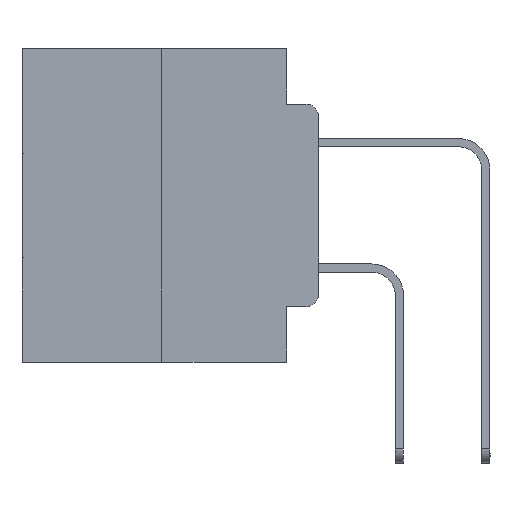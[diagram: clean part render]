
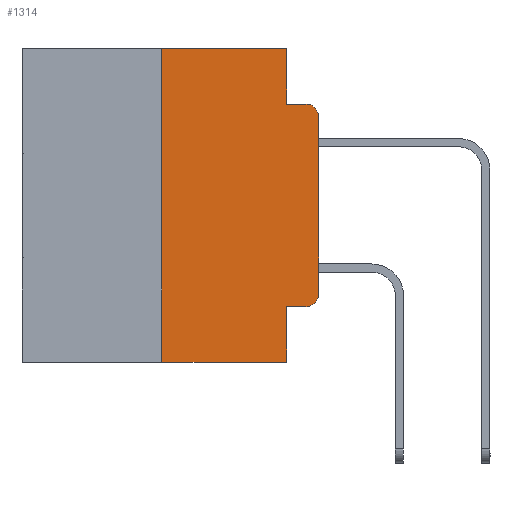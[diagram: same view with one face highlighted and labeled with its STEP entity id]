
A CAD part, left-side view. The second image highlights one B-rep face of the part: STEP entity #1314.
In plain terms, the highlighted planar face has unit normal (-1, 0, 0).
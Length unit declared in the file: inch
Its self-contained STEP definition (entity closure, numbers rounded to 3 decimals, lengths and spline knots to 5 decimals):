
#686 = VECTOR ( 'NONE', #9635, 39.37008 ) ;
#1071 = EDGE_LOOP ( 'NONE', ( #18724, #27887, #17250, #8662, #7042, #16825, #24293, #7595, #14695, #12281 ) ) ;
#1314 = ADVANCED_FACE ( 'NONE', ( #29013 ), #4517, .F. ) ;
#1382 = VECTOR ( 'NONE', #10721, 39.37008 ) ;
#1908 = CARTESIAN_POINT ( 'NONE',  ( 0., 0.02, -0.3915 ) ) ;
#2216 = DIRECTION ( 'NONE',  ( 0., 0., -1. ) ) ;
#2251 = VERTEX_POINT ( 'NONE', #7929 ) ;
#2309 = CARTESIAN_POINT ( 'NONE',  ( 0., 0.25, 0. ) ) ;
#2750 = EDGE_CURVE ( 'NONE', #13544, #15908, #11749, .T. ) ;
#2816 = VERTEX_POINT ( 'NONE', #22312 ) ;
#3006 = DIRECTION ( 'NONE',  ( 0., 0., 1. ) ) ;
#3045 = EDGE_CURVE ( 'NONE', #2816, #2251, #11029, .T. ) ;
#4202 = AXIS2_PLACEMENT_3D ( 'NONE', #1908, #6905, #8950 ) ;
#4517 = PLANE ( 'NONE',  #7784 ) ;
#4700 = EDGE_CURVE ( 'NONE', #25344, #2816, #19613, .T. ) ;
#5399 = EDGE_CURVE ( 'NONE', #25885, #25344, #24340, .T. ) ;
#5904 = CARTESIAN_POINT ( 'NONE',  ( 0., 0.473, -0.5 ) ) ;
#6094 = EDGE_CURVE ( 'NONE', #20233, #19819, #14853, .T. ) ;
#6693 = CARTESIAN_POINT ( 'NONE',  ( 0., 0.051, 0. ) ) ;
#6724 = CARTESIAN_POINT ( 'NONE',  ( 0., 0.473, 0. ) ) ;
#6905 = DIRECTION ( 'NONE',  ( -1., 0., 0. ) ) ;
#6914 = LINE ( 'NONE', #5904, #17869 ) ;
#7042 = ORIENTED_EDGE ( 'NONE', *, *, #2750, .F. ) ;
#7595 = ORIENTED_EDGE ( 'NONE', *, *, #6094, .F. ) ;
#7784 = AXIS2_PLACEMENT_3D ( 'NONE', #6724, #20775, #25341 ) ;
#7929 = CARTESIAN_POINT ( 'NONE',  ( 0., 0.02, -0.0885 ) ) ;
#8468 = DIRECTION ( 'NONE',  ( 0., -1., 0. ) ) ;
#8662 = ORIENTED_EDGE ( 'NONE', *, *, #24533, .F. ) ;
#8950 = DIRECTION ( 'NONE',  ( 0., 0., -1. ) ) ;
#9635 = DIRECTION ( 'NONE',  ( 0., 0., -1. ) ) ;
#9877 = CARTESIAN_POINT ( 'NONE',  ( 0., 0., 0. ) ) ;
#9967 = EDGE_CURVE ( 'NONE', #13667, #19819, #6914, .T. ) ;
#10721 = DIRECTION ( 'NONE',  ( 0., -1., 0. ) ) ;
#11029 = CIRCLE ( 'NONE', #21854, 0.02 ) ;
#11208 = CARTESIAN_POINT ( 'NONE',  ( 0., 0.25, 0. ) ) ;
#11445 = CARTESIAN_POINT ( 'NONE',  ( 0., 0.02, -0.1085 ) ) ;
#11591 = DIRECTION ( 'NONE',  ( 0., 0., -1. ) ) ;
#11749 = LINE ( 'NONE', #13150, #29911 ) ;
#12281 = ORIENTED_EDGE ( 'NONE', *, *, #5399, .T. ) ;
#12446 = CARTESIAN_POINT ( 'NONE',  ( 0., 0., -0.3915 ) ) ;
#12686 = LINE ( 'NONE', #2309, #16325 ) ;
#13041 = DIRECTION ( 'NONE',  ( 0., -1., 0. ) ) ;
#13150 = CARTESIAN_POINT ( 'NONE',  ( 0., 0.473, 0. ) ) ;
#13361 = EDGE_CURVE ( 'NONE', #14146, #2251, #14140, .T. ) ;
#13544 = VERTEX_POINT ( 'NONE', #11208 ) ;
#13667 = VERTEX_POINT ( 'NONE', #16709 ) ;
#14139 = CARTESIAN_POINT ( 'NONE',  ( 0., 0.051, 0. ) ) ;
#14140 = LINE ( 'NONE', #20375, #29391 ) ;
#14146 = VERTEX_POINT ( 'NONE', #16875 ) ;
#14429 = CARTESIAN_POINT ( 'NONE',  ( 0., 0.051, 0. ) ) ;
#14695 = ORIENTED_EDGE ( 'NONE', *, *, #21782, .T. ) ;
#14853 = LINE ( 'NONE', #14429, #686 ) ;
#15908 = VERTEX_POINT ( 'NONE', #6693 ) ;
#15966 = CARTESIAN_POINT ( 'NONE',  ( 0., 0.051, -0.5 ) ) ;
#16325 = VECTOR ( 'NONE', #19064, 39.37008 ) ;
#16709 = CARTESIAN_POINT ( 'NONE',  ( 0., 0.25, -0.5 ) ) ;
#16717 = EDGE_CURVE ( 'NONE', #13667, #13544, #12686, .T. ) ;
#16811 = VECTOR ( 'NONE', #11591, 39.37008 ) ;
#16825 = ORIENTED_EDGE ( 'NONE', *, *, #16717, .F. ) ;
#16875 = CARTESIAN_POINT ( 'NONE',  ( 0., 0.051, -0.0885 ) ) ;
#17250 = ORIENTED_EDGE ( 'NONE', *, *, #13361, .F. ) ;
#17869 = VECTOR ( 'NONE', #27138, 39.37008 ) ;
#18724 = ORIENTED_EDGE ( 'NONE', *, *, #4700, .T. ) ;
#18787 = LINE ( 'NONE', #29493, #1382 ) ;
#19064 = DIRECTION ( 'NONE',  ( 0., 0., 1. ) ) ;
#19613 = LINE ( 'NONE', #9877, #26169 ) ;
#19819 = VERTEX_POINT ( 'NONE', #15966 ) ;
#20233 = VERTEX_POINT ( 'NONE', #22740 ) ;
#20375 = CARTESIAN_POINT ( 'NONE',  ( 0., 0.051, -0.0885 ) ) ;
#20775 = DIRECTION ( 'NONE',  ( 1., 0., 0. ) ) ;
#21434 = CARTESIAN_POINT ( 'NONE',  ( 0., 0.02, -0.4115 ) ) ;
#21782 = EDGE_CURVE ( 'NONE', #20233, #25885, #18787, .T. ) ;
#21854 = AXIS2_PLACEMENT_3D ( 'NONE', #11445, #27715, #2216 ) ;
#22312 = CARTESIAN_POINT ( 'NONE',  ( 0., 0., -0.1085 ) ) ;
#22740 = CARTESIAN_POINT ( 'NONE',  ( 0., 0.051, -0.4115 ) ) ;
#24293 = ORIENTED_EDGE ( 'NONE', *, *, #9967, .T. ) ;
#24340 = CIRCLE ( 'NONE', #4202, 0.02 ) ;
#24533 = EDGE_CURVE ( 'NONE', #15908, #14146, #28050, .T. ) ;
#25341 = DIRECTION ( 'NONE',  ( 0., 0., -1. ) ) ;
#25344 = VERTEX_POINT ( 'NONE', #12446 ) ;
#25885 = VERTEX_POINT ( 'NONE', #21434 ) ;
#26169 = VECTOR ( 'NONE', #3006, 39.37008 ) ;
#27138 = DIRECTION ( 'NONE',  ( 0., -1., 0. ) ) ;
#27715 = DIRECTION ( 'NONE',  ( -1., 0., 0. ) ) ;
#27887 = ORIENTED_EDGE ( 'NONE', *, *, #3045, .T. ) ;
#28050 = LINE ( 'NONE', #14139, #16811 ) ;
#29013 = FACE_OUTER_BOUND ( 'NONE', #1071, .T. ) ;
#29391 = VECTOR ( 'NONE', #8468, 39.37008 ) ;
#29493 = CARTESIAN_POINT ( 'NONE',  ( 0., 0.051, -0.4115 ) ) ;
#29911 = VECTOR ( 'NONE', #13041, 39.37008 ) ;
